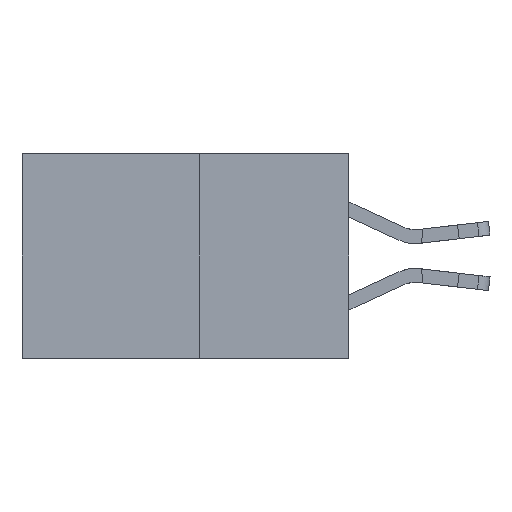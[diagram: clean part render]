
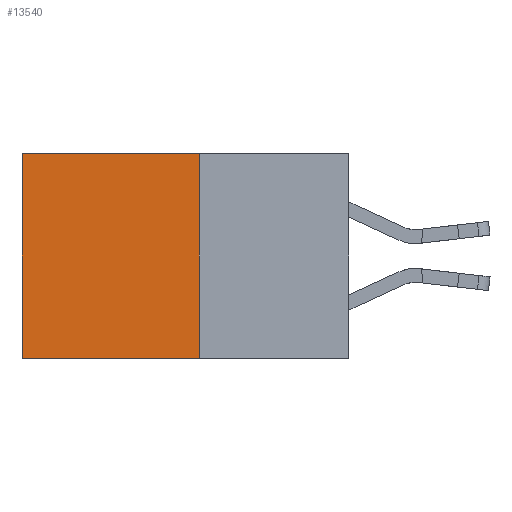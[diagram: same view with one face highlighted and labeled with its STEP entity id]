
A CAD part, left-side view. The second image highlights one B-rep face of the part: STEP entity #13540.
In plain terms, the highlighted planar face has unit normal (-1, 0, 0).
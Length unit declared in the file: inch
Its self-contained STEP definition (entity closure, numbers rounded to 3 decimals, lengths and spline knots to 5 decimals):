
#13 = ORIENTED_EDGE ( 'NONE', *, *, #5655, .T. ) ;
#102 = ORIENTED_EDGE ( 'NONE', *, *, #5292, .F. ) ;
#149 = LINE ( 'NONE', #8007, #2744 ) ;
#306 = ORIENTED_EDGE ( 'NONE', *, *, #2021, .T. ) ;
#1072 = CARTESIAN_POINT ( 'NONE',  ( 0.277, 0.59, -0.37 ) ) ;
#1201 = CARTESIAN_POINT ( 'NONE',  ( 0.277, 0.27, -0.37 ) ) ;
#2021 = EDGE_CURVE ( 'NONE', #12943, #9195, #149, .T. ) ;
#2262 = VECTOR ( 'NONE', #10799, 39.37008 ) ;
#2429 = DIRECTION ( 'NONE',  ( 0., 1., 0. ) ) ;
#2744 = VECTOR ( 'NONE', #5740, 39.37008 ) ;
#2765 = AXIS2_PLACEMENT_3D ( 'NONE', #1201, #11075, #4574 ) ;
#2805 = CARTESIAN_POINT ( 'NONE',  ( 0.277, 0.27, 0. ) ) ;
#2966 = VECTOR ( 'NONE', #10609, 39.37008 ) ;
#3024 = CARTESIAN_POINT ( 'NONE',  ( 0.277, 0.27, -0.37 ) ) ;
#3329 = VECTOR ( 'NONE', #2429, 39.37008 ) ;
#3490 = PLANE ( 'NONE',  #2765 ) ;
#3497 = ORIENTED_EDGE ( 'NONE', *, *, #9008, .F. ) ;
#4181 = CARTESIAN_POINT ( 'NONE',  ( 0.277, 0.27, 0. ) ) ;
#4574 = DIRECTION ( 'NONE',  ( 0., 0., -1. ) ) ;
#4645 = CARTESIAN_POINT ( 'NONE',  ( 0.277, 0.59, 0. ) ) ;
#4698 = VERTEX_POINT ( 'NONE', #5159 ) ;
#5159 = CARTESIAN_POINT ( 'NONE',  ( 0.277, 0.27, -0.37 ) ) ;
#5292 = EDGE_CURVE ( 'NONE', #5574, #4698, #13328, .T. ) ;
#5529 = LINE ( 'NONE', #3024, #2966 ) ;
#5574 = VERTEX_POINT ( 'NONE', #4181 ) ;
#5655 = EDGE_CURVE ( 'NONE', #5574, #12943, #6241, .T. ) ;
#5740 = DIRECTION ( 'NONE',  ( 0., 0., -1. ) ) ;
#5985 = EDGE_LOOP ( 'NONE', ( #306, #3497, #102, #13 ) ) ;
#6241 = LINE ( 'NONE', #2805, #3329 ) ;
#8007 = CARTESIAN_POINT ( 'NONE',  ( 0.277, 0.59, -0.37 ) ) ;
#8297 = FACE_OUTER_BOUND ( 'NONE', #5985, .T. ) ;
#9008 = EDGE_CURVE ( 'NONE', #4698, #9195, #5529, .T. ) ;
#9195 = VERTEX_POINT ( 'NONE', #1072 ) ;
#10508 = CARTESIAN_POINT ( 'NONE',  ( 0.277, 0.27, -0.37 ) ) ;
#10609 = DIRECTION ( 'NONE',  ( 0., 1., 0. ) ) ;
#10799 = DIRECTION ( 'NONE',  ( 0., 0., -1. ) ) ;
#11075 = DIRECTION ( 'NONE',  ( 1., 0., 0. ) ) ;
#12943 = VERTEX_POINT ( 'NONE', #4645 ) ;
#13328 = LINE ( 'NONE', #10508, #2262 ) ;
#13540 = ADVANCED_FACE ( 'NONE', ( #8297 ), #3490, .F. ) ;
